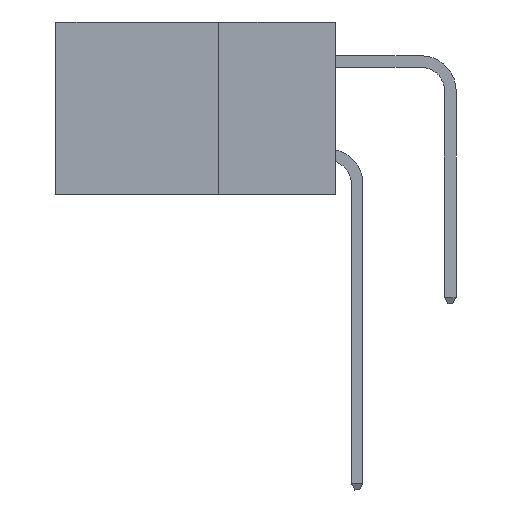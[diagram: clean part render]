
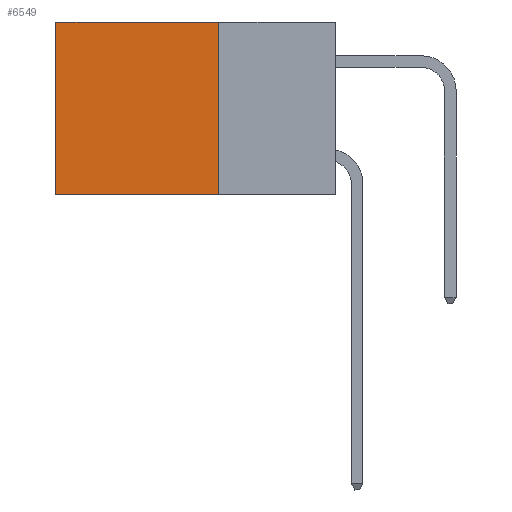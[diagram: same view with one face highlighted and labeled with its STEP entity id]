
A CAD part, left-side view. The second image highlights one B-rep face of the part: STEP entity #6549.
In plain terms, the highlighted planar face has unit normal (-1, 0, 0).
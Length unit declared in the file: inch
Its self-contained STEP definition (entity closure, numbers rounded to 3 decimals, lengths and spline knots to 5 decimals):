
#275 = DIRECTION ( 'NONE',  ( 0., 0., -1. ) ) ;
#2826 = CARTESIAN_POINT ( 'NONE',  ( 0.2875, 0.25, -0.37 ) ) ;
#3889 = AXIS2_PLACEMENT_3D ( 'NONE', #33951, #21551, #34765 ) ;
#4094 = VECTOR ( 'NONE', #5389, 39.37008 ) ;
#5389 = DIRECTION ( 'NONE',  ( 0., 1., 0. ) ) ;
#6300 = LINE ( 'NONE', #18935, #34819 ) ;
#6549 = ADVANCED_FACE ( 'NONE', ( #22156 ), #9528, .F. ) ;
#9528 = PLANE ( 'NONE',  #3889 ) ;
#10177 = DIRECTION ( 'NONE',  ( 0., 0., -1. ) ) ;
#12660 = EDGE_LOOP ( 'NONE', ( #24912, #21746, #16794, #25630 ) ) ;
#14212 = VECTOR ( 'NONE', #275, 39.37008 ) ;
#15339 = CARTESIAN_POINT ( 'NONE',  ( 0.2875, 0.25, -0.37 ) ) ;
#15525 = CARTESIAN_POINT ( 'NONE',  ( 0.2875, 0.6, 0. ) ) ;
#16029 = VERTEX_POINT ( 'NONE', #15525 ) ;
#16794 = ORIENTED_EDGE ( 'NONE', *, *, #18342, .F. ) ;
#18342 = EDGE_CURVE ( 'NONE', #33137, #25840, #19550, .T. ) ;
#18935 = CARTESIAN_POINT ( 'NONE',  ( 0.2875, 0.25, 0. ) ) ;
#19516 = VERTEX_POINT ( 'NONE', #40132 ) ;
#19550 = LINE ( 'NONE', #32144, #14212 ) ;
#21551 = DIRECTION ( 'NONE',  ( 1., 0., 0. ) ) ;
#21730 = LINE ( 'NONE', #15339, #4094 ) ;
#21746 = ORIENTED_EDGE ( 'NONE', *, *, #34789, .F. ) ;
#22156 = FACE_OUTER_BOUND ( 'NONE', #12660, .T. ) ;
#24869 = CARTESIAN_POINT ( 'NONE',  ( 0.2875, 0.25, 0. ) ) ;
#24912 = ORIENTED_EDGE ( 'NONE', *, *, #34621, .T. ) ;
#25630 = ORIENTED_EDGE ( 'NONE', *, *, #27553, .T. ) ;
#25840 = VERTEX_POINT ( 'NONE', #2826 ) ;
#27553 = EDGE_CURVE ( 'NONE', #33137, #16029, #6300, .T. ) ;
#28643 = DIRECTION ( 'NONE',  ( 0., 1., 0. ) ) ;
#32084 = LINE ( 'NONE', #38098, #35738 ) ;
#32144 = CARTESIAN_POINT ( 'NONE',  ( 0.2875, 0.25, 0. ) ) ;
#33137 = VERTEX_POINT ( 'NONE', #24869 ) ;
#33951 = CARTESIAN_POINT ( 'NONE',  ( 0.2875, 0.25, 0. ) ) ;
#34621 = EDGE_CURVE ( 'NONE', #16029, #19516, #32084, .T. ) ;
#34765 = DIRECTION ( 'NONE',  ( 0., 0., -1. ) ) ;
#34789 = EDGE_CURVE ( 'NONE', #25840, #19516, #21730, .T. ) ;
#34819 = VECTOR ( 'NONE', #28643, 39.37008 ) ;
#35738 = VECTOR ( 'NONE', #10177, 39.37008 ) ;
#38098 = CARTESIAN_POINT ( 'NONE',  ( 0.2875, 0.6, 0. ) ) ;
#40132 = CARTESIAN_POINT ( 'NONE',  ( 0.2875, 0.6, -0.37 ) ) ;
